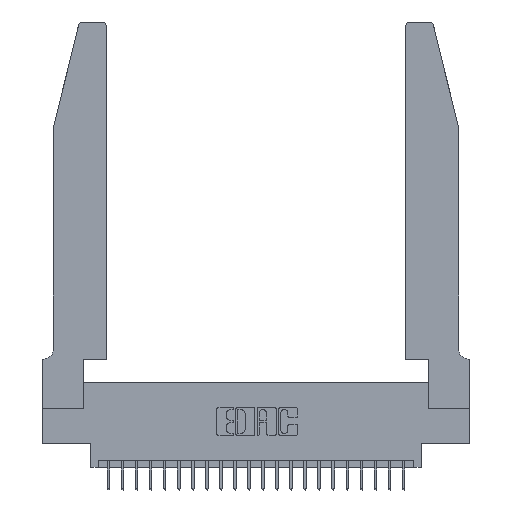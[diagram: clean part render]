
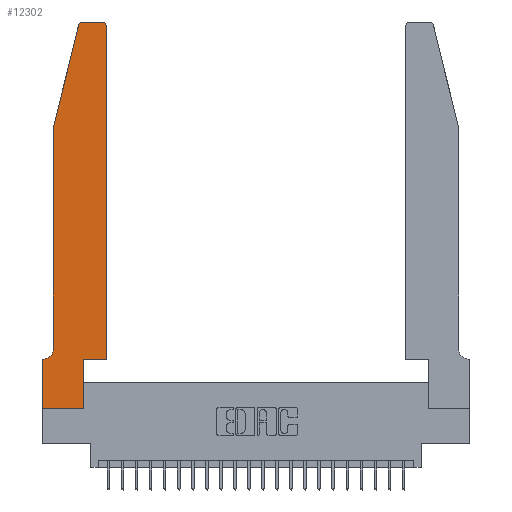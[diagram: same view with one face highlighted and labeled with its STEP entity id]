
A CAD part, top view. The second image highlights one B-rep face of the part: STEP entity #12302.
In plain terms, the highlighted planar face has unit normal (0, 0, 1).
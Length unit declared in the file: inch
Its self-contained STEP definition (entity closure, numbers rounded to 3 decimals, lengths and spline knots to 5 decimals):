
#38 = VERTEX_POINT ( 'NONE', #17576 ) ;
#481 = EDGE_CURVE ( 'NONE', #9786, #19952, #11070, .T. ) ;
#553 = DIRECTION ( 'NONE',  ( 0., 0., -1. ) ) ;
#1832 = VECTOR ( 'NONE', #13007, 39.37008 ) ;
#1835 = ORIENTED_EDGE ( 'NONE', *, *, #23658, .T. ) ;
#1985 = LINE ( 'NONE', #19852, #11710 ) ;
#2097 = VERTEX_POINT ( 'NONE', #2404 ) ;
#2151 = CARTESIAN_POINT ( 'NONE',  ( 0.4505, 0.35, 0.37 ) ) ;
#2404 = CARTESIAN_POINT ( 'NONE',  ( 0.284, 2.75, 0.37 ) ) ;
#2500 = CARTESIAN_POINT ( 'NONE',  ( 0., 0., 0.37 ) ) ;
#2872 = EDGE_CURVE ( 'NONE', #10344, #5750, #10341, .T. ) ;
#3089 = EDGE_CURVE ( 'NONE', #5507, #15751, #20178, .T. ) ;
#3097 = LINE ( 'NONE', #24407, #1832 ) ;
#3473 = DIRECTION ( 'NONE',  ( 1., 0., 0. ) ) ;
#3774 = VERTEX_POINT ( 'NONE', #7330 ) ;
#4121 = DIRECTION ( 'NONE',  ( 0., 1., 0. ) ) ;
#4218 = CARTESIAN_POINT ( 'NONE',  ( 0.25487, 2.72718, 0.37 ) ) ;
#4295 = VERTEX_POINT ( 'NONE', #14548 ) ;
#4451 = DIRECTION ( 'NONE',  ( 1., 0., 0. ) ) ;
#4573 = VECTOR ( 'NONE', #12607, 39.37008 ) ;
#4660 = ORIENTED_EDGE ( 'NONE', *, *, #24707, .T. ) ;
#5104 = LINE ( 'NONE', #16808, #19822 ) ;
#5196 = ORIENTED_EDGE ( 'NONE', *, *, #7746, .T. ) ;
#5242 = ORIENTED_EDGE ( 'NONE', *, *, #8818, .T. ) ;
#5507 = VERTEX_POINT ( 'NONE', #14741 ) ;
#5533 = EDGE_LOOP ( 'NONE', ( #16922, #5196, #21124, #1835, #13374, #6401, #5242, #10996, #17602, #4660, #22974, #9551 ) ) ;
#5750 = VERTEX_POINT ( 'NONE', #17223 ) ;
#5813 = VERTEX_POINT ( 'NONE', #19808 ) ;
#5908 = VECTOR ( 'NONE', #7994, 39.37008 ) ;
#6348 = AXIS2_PLACEMENT_3D ( 'NONE', #20037, #8608, #21970 ) ;
#6401 = ORIENTED_EDGE ( 'NONE', *, *, #2872, .T. ) ;
#6772 = DIRECTION ( 'NONE',  ( 0., -1., 0. ) ) ;
#6870 = CARTESIAN_POINT ( 'NONE',  ( 0.2865, 0.35, 0.37 ) ) ;
#7330 = CARTESIAN_POINT ( 'NONE',  ( 0.4205, 2.75, 0.37 ) ) ;
#7746 = EDGE_CURVE ( 'NONE', #2097, #9786, #8281, .T. ) ;
#7994 = DIRECTION ( 'NONE',  ( -0.239, -0.971, 0. ) ) ;
#8281 = CIRCLE ( 'NONE', #6348, 0.03 ) ;
#8393 = AXIS2_PLACEMENT_3D ( 'NONE', #18759, #15003, #3473 ) ;
#8608 = DIRECTION ( 'NONE',  ( 0., 0., 1. ) ) ;
#8710 = VERTEX_POINT ( 'NONE', #23787 ) ;
#8818 = EDGE_CURVE ( 'NONE', #5750, #38, #9254, .T. ) ;
#9115 = LINE ( 'NONE', #2151, #23137 ) ;
#9254 = LINE ( 'NONE', #20210, #18803 ) ;
#9551 = ORIENTED_EDGE ( 'NONE', *, *, #13531, .T. ) ;
#9600 = DIRECTION ( 'NONE',  ( 0., 0., 1. ) ) ;
#9786 = VERTEX_POINT ( 'NONE', #4218 ) ;
#10341 = LINE ( 'NONE', #20186, #4573 ) ;
#10342 = DIRECTION ( 'NONE',  ( 1., 0., 0. ) ) ;
#10344 = VERTEX_POINT ( 'NONE', #23479 ) ;
#10996 = ORIENTED_EDGE ( 'NONE', *, *, #14236, .T. ) ;
#11070 = LINE ( 'NONE', #19971, #5908 ) ;
#11710 = VECTOR ( 'NONE', #10342, 39.37008 ) ;
#12188 = CARTESIAN_POINT ( 'NONE',  ( 0.0055, 0.42, 0.37 ) ) ;
#12302 = ADVANCED_FACE ( 'NONE', ( #17067 ), #22591, .T. ) ;
#12320 = EDGE_CURVE ( 'NONE', #4295, #8710, #9115, .T. ) ;
#12607 = DIRECTION ( 'NONE',  ( -1., 0., 0. ) ) ;
#13007 = DIRECTION ( 'NONE',  ( -1., 0., 0. ) ) ;
#13187 = DIRECTION ( 'NONE',  ( 0., 1., 0. ) ) ;
#13374 = ORIENTED_EDGE ( 'NONE', *, *, #18642, .T. ) ;
#13531 = EDGE_CURVE ( 'NONE', #8710, #3774, #23973, .T. ) ;
#14119 = DIRECTION ( 'NONE',  ( -1., 0., 0. ) ) ;
#14236 = EDGE_CURVE ( 'NONE', #38, #5507, #15278, .T. ) ;
#14548 = CARTESIAN_POINT ( 'NONE',  ( 0.4505, 0.35, 0.37 ) ) ;
#14741 = CARTESIAN_POINT ( 'NONE',  ( 0.2865, 0., 0.37 ) ) ;
#15003 = DIRECTION ( 'NONE',  ( 0., 0., 1. ) ) ;
#15278 = LINE ( 'NONE', #2500, #18570 ) ;
#15751 = VERTEX_POINT ( 'NONE', #6870 ) ;
#16808 = CARTESIAN_POINT ( 'NONE',  ( 0.0755, 2., 0.37 ) ) ;
#16828 = AXIS2_PLACEMENT_3D ( 'NONE', #12188, #553, #14119 ) ;
#16922 = ORIENTED_EDGE ( 'NONE', *, *, #17714, .T. ) ;
#17067 = FACE_OUTER_BOUND ( 'NONE', #5533, .T. ) ;
#17223 = CARTESIAN_POINT ( 'NONE',  ( 0., 0.35, 0.37 ) ) ;
#17576 = CARTESIAN_POINT ( 'NONE',  ( 0., 0., 0.37 ) ) ;
#17602 = ORIENTED_EDGE ( 'NONE', *, *, #3089, .T. ) ;
#17714 = EDGE_CURVE ( 'NONE', #3774, #2097, #3097, .T. ) ;
#18570 = VECTOR ( 'NONE', #4451, 39.37008 ) ;
#18642 = EDGE_CURVE ( 'NONE', #5813, #10344, #24332, .T. ) ;
#18735 = DIRECTION ( 'NONE',  ( 0., -1., 0. ) ) ;
#18759 = CARTESIAN_POINT ( 'NONE',  ( 0., 0.35, 0.37 ) ) ;
#18803 = VECTOR ( 'NONE', #6772, 39.37008 ) ;
#18845 = AXIS2_PLACEMENT_3D ( 'NONE', #21040, #9600, #22941 ) ;
#19808 = CARTESIAN_POINT ( 'NONE',  ( 0.0755, 0.42, 0.37 ) ) ;
#19822 = VECTOR ( 'NONE', #18735, 39.37008 ) ;
#19852 = CARTESIAN_POINT ( 'NONE',  ( 0.4505, 0.35, 0.37 ) ) ;
#19952 = VERTEX_POINT ( 'NONE', #19993 ) ;
#19971 = CARTESIAN_POINT ( 'NONE',  ( 0.0755, 2., 0.37 ) ) ;
#19993 = CARTESIAN_POINT ( 'NONE',  ( 0.0755, 2., 0.37 ) ) ;
#20037 = CARTESIAN_POINT ( 'NONE',  ( 0.284, 2.72, 0.37 ) ) ;
#20178 = LINE ( 'NONE', #22678, #20788 ) ;
#20186 = CARTESIAN_POINT ( 'NONE',  ( 0.0755, 0.35, 0.37 ) ) ;
#20210 = CARTESIAN_POINT ( 'NONE',  ( 0., 0., 0.37 ) ) ;
#20788 = VECTOR ( 'NONE', #13187, 39.37008 ) ;
#21040 = CARTESIAN_POINT ( 'NONE',  ( 0.4205, 2.72, 0.37 ) ) ;
#21124 = ORIENTED_EDGE ( 'NONE', *, *, #481, .T. ) ;
#21970 = DIRECTION ( 'NONE',  ( 1., 0., 0. ) ) ;
#22591 = PLANE ( 'NONE',  #8393 ) ;
#22678 = CARTESIAN_POINT ( 'NONE',  ( 0.2865, 0.35, 0.37 ) ) ;
#22941 = DIRECTION ( 'NONE',  ( 1., 0., 0. ) ) ;
#22974 = ORIENTED_EDGE ( 'NONE', *, *, #12320, .T. ) ;
#23137 = VECTOR ( 'NONE', #4121, 39.37008 ) ;
#23479 = CARTESIAN_POINT ( 'NONE',  ( 0.0055, 0.35, 0.37 ) ) ;
#23658 = EDGE_CURVE ( 'NONE', #19952, #5813, #5104, .T. ) ;
#23787 = CARTESIAN_POINT ( 'NONE',  ( 0.4505, 2.72, 0.37 ) ) ;
#23973 = CIRCLE ( 'NONE', #18845, 0.03 ) ;
#24332 = CIRCLE ( 'NONE', #16828, 0.07 ) ;
#24407 = CARTESIAN_POINT ( 'NONE',  ( 0.2605, 2.75, 0.37 ) ) ;
#24707 = EDGE_CURVE ( 'NONE', #15751, #4295, #1985, .T. ) ;
